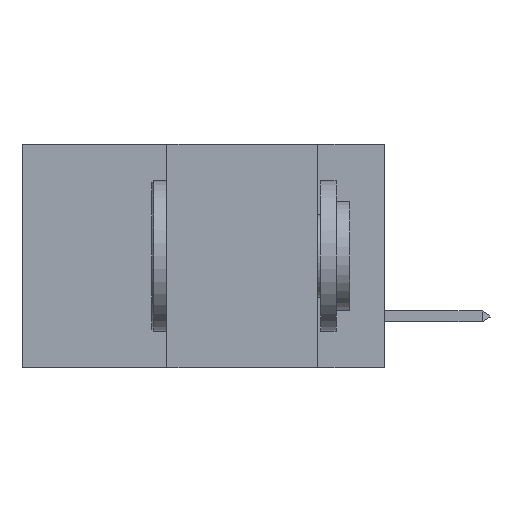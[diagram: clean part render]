
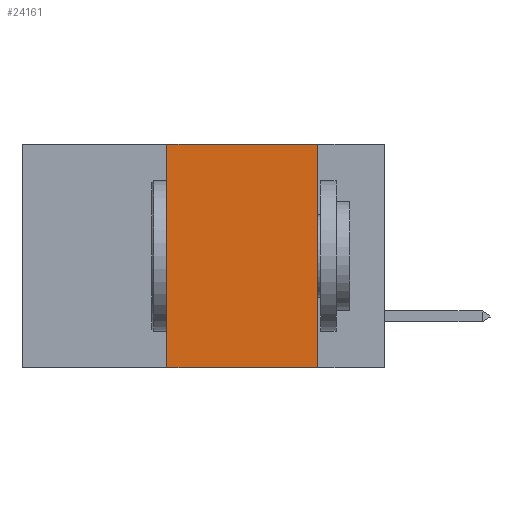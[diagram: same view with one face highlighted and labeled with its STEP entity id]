
A CAD part, left-side view. The second image highlights one B-rep face of the part: STEP entity #24161.
In plain terms, the highlighted planar face has unit normal (-1, 0, 0).
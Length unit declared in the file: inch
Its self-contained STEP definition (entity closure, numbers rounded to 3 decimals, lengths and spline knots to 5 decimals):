
#55 = LINE ( 'NONE', #12944, #12922 ) ;
#661 = VECTOR ( 'NONE', #16557, 39.37008 ) ;
#4103 = EDGE_CURVE ( 'NONE', #29346, #16993, #9868, .T. ) ;
#4919 = ORIENTED_EDGE ( 'NONE', *, *, #17131, .T. ) ;
#6850 = CARTESIAN_POINT ( 'NONE',  ( 0., 0.6, -0.37 ) ) ;
#7140 = EDGE_CURVE ( 'NONE', #14647, #29346, #55, .T. ) ;
#8819 = FACE_OUTER_BOUND ( 'NONE', #27915, .T. ) ;
#8871 = DIRECTION ( 'NONE',  ( 0., 0., 1. ) ) ;
#9868 = LINE ( 'NONE', #16475, #12904 ) ;
#10584 = CARTESIAN_POINT ( 'NONE',  ( 0., 0.11, -0.37 ) ) ;
#10872 = DIRECTION ( 'NONE',  ( 0., 0., -1. ) ) ;
#12682 = ORIENTED_EDGE ( 'NONE', *, *, #7140, .F. ) ;
#12904 = VECTOR ( 'NONE', #10872, 39.37008 ) ;
#12922 = VECTOR ( 'NONE', #22771, 39.37008 ) ;
#12944 = CARTESIAN_POINT ( 'NONE',  ( 0., 0.6, 0. ) ) ;
#13959 = ORIENTED_EDGE ( 'NONE', *, *, #4103, .F. ) ;
#14647 = VERTEX_POINT ( 'NONE', #31082 ) ;
#15295 = DIRECTION ( 'NONE',  ( 1., 0., 0. ) ) ;
#16257 = CARTESIAN_POINT ( 'NONE',  ( 0., 0.36, 0. ) ) ;
#16475 = CARTESIAN_POINT ( 'NONE',  ( 0., 0.11, 0. ) ) ;
#16557 = DIRECTION ( 'NONE',  ( 0., -1., 0. ) ) ;
#16993 = VERTEX_POINT ( 'NONE', #10584 ) ;
#17131 = EDGE_CURVE ( 'NONE', #24894, #16993, #24446, .T. ) ;
#17841 = PLANE ( 'NONE',  #20928 ) ;
#19275 = ORIENTED_EDGE ( 'NONE', *, *, #23757, .F. ) ;
#20367 = DIRECTION ( 'NONE',  ( 0., 0., -1. ) ) ;
#20928 = AXIS2_PLACEMENT_3D ( 'NONE', #27726, #15295, #20367 ) ;
#21276 = CARTESIAN_POINT ( 'NONE',  ( 0., 0.11, 0. ) ) ;
#21277 = VECTOR ( 'NONE', #8871, 39.37008 ) ;
#22771 = DIRECTION ( 'NONE',  ( 0., -1., 0. ) ) ;
#23757 = EDGE_CURVE ( 'NONE', #24894, #14647, #30353, .T. ) ;
#24161 = ADVANCED_FACE ( 'NONE', ( #8819 ), #17841, .F. ) ;
#24446 = LINE ( 'NONE', #6850, #661 ) ;
#24894 = VERTEX_POINT ( 'NONE', #27680 ) ;
#27680 = CARTESIAN_POINT ( 'NONE',  ( 0., 0.36, -0.37 ) ) ;
#27726 = CARTESIAN_POINT ( 'NONE',  ( 0., 0.6, 0. ) ) ;
#27915 = EDGE_LOOP ( 'NONE', ( #13959, #12682, #19275, #4919 ) ) ;
#29346 = VERTEX_POINT ( 'NONE', #21276 ) ;
#30353 = LINE ( 'NONE', #16257, #21277 ) ;
#31082 = CARTESIAN_POINT ( 'NONE',  ( 0., 0.36, 0. ) ) ;
